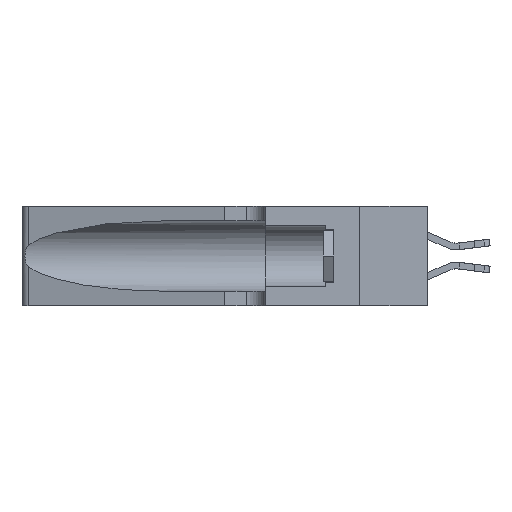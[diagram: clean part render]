
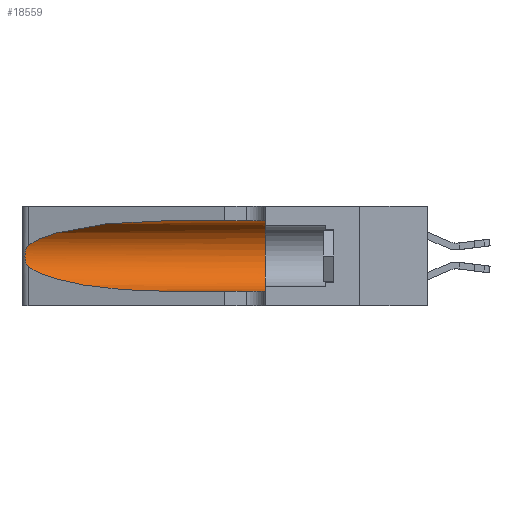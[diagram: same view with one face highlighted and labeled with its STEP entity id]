
A CAD part, left-side view. The second image highlights one B-rep face of the part: STEP entity #18559.
In plain terms, the highlighted cylindrical face has radius 3.308 mm (diameter 6.617 mm), a partial arc.
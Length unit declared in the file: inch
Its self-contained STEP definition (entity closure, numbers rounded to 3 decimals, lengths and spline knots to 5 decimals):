
#207 =( BOUNDED_CURVE ( )  B_SPLINE_CURVE ( 3, ( #34187, #9780, #20865, #4327 ),
 .UNSPECIFIED., .F., .F. ) 
 B_SPLINE_CURVE_WITH_KNOTS ( ( 4, 4 ),
 ( 1.5708, 2.84003 ),
 .UNSPECIFIED. ) 
 CURVE ( )  GEOMETRIC_REPRESENTATION_ITEM ( )  RATIONAL_B_SPLINE_CURVE ( ( 1., 0.87, 0.87, 1. ) ) 
 REPRESENTATION_ITEM ( '' )  );
#319 = LINE ( 'NONE', #3839, #20678 ) ;
#564 = CYLINDRICAL_SURFACE ( 'NONE', #26743, 0.13025 ) ;
#777 = VERTEX_POINT ( 'NONE', #2038 ) ;
#1110 = CARTESIAN_POINT ( 'NONE',  ( 0.26075, 1.23896, 0.19203 ) ) ;
#1728 = EDGE_CURVE ( 'NONE', #10739, #4429, #319, .T. ) ;
#2038 = CARTESIAN_POINT ( 'NONE',  ( 0.25487, 1.22718, 0.14631 ) ) ;
#3839 = CARTESIAN_POINT ( 'NONE',  ( 0.1305, 1.61858, 0.31525 ) ) ;
#3935 = CARTESIAN_POINT ( 'NONE',  ( 0.26017, 1.23833, 0.17102 ) ) ;
#4327 = CARTESIAN_POINT ( 'NONE',  ( 0.25487, 1.22718, 0.22369 ) ) ;
#4376 = CARTESIAN_POINT ( 'NONE',  ( 0.1305, 0.35, 0.05475 ) ) ;
#4429 = VERTEX_POINT ( 'NONE', #34264 ) ;
#4740 = CARTESIAN_POINT ( 'NONE',  ( 0.1305, 0.72297, 0.31525 ) ) ;
#5566 = CIRCLE ( 'NONE', #7672, 0.13025 ) ;
#6512 = DIRECTION ( 'NONE',  ( 0., -1., 0. ) ) ;
#6612 = CARTESIAN_POINT ( 'NONE',  ( 0.25555, 1.22994, 0.2215 ) ) ;
#6734 = CARTESIAN_POINT ( 'NONE',  ( 0.25789, 1.23486, 0.15765 ) ) ;
#7672 = AXIS2_PLACEMENT_3D ( 'NONE', #27172, #10840, #29888 ) ;
#7956 = CARTESIAN_POINT ( 'NONE',  ( 0.1305, 0.72297, 0.05475 ) ) ;
#8739 = VERTEX_POINT ( 'NONE', #25082 ) ;
#9367 = ORIENTED_EDGE ( 'NONE', *, *, #26774, .T. ) ;
#9428 = CARTESIAN_POINT ( 'NONE',  ( 0.1305, 0.72297, 0.05475 ) ) ;
#9519 = CARTESIAN_POINT ( 'NONE',  ( 0.25555, 1.22993, 0.14849 ) ) ;
#9780 = CARTESIAN_POINT ( 'NONE',  ( 0.18966, 0.96281, 0.31525 ) ) ;
#10739 = VERTEX_POINT ( 'NONE', #4740 ) ;
#10840 = DIRECTION ( 'NONE',  ( 0., 1., 0. ) ) ;
#11029 = LINE ( 'NONE', #22103, #25579 ) ;
#11412 = ORIENTED_EDGE ( 'NONE', *, *, #1728, .F. ) ;
#11451 = EDGE_LOOP ( 'NONE', ( #9367, #31678, #34146, #22900, #24126, #11412 ) ) ;
#11585 = DIRECTION ( 'NONE',  ( 0., -1., 0. ) ) ;
#12893 = EDGE_CURVE ( 'NONE', #34045, #18860, #11029, .T. ) ;
#14989 = CARTESIAN_POINT ( 'NONE',  ( 0.25787, 1.23484, 0.2124 ) ) ;
#15813 = B_SPLINE_CURVE_WITH_KNOTS ( 'NONE', 3,
 ( #23095, #6612, #31202, #14989, #33924, #17776, #1110, #20496, #3935, #23217, #6734, #25928, #9519, #28628 ),
 .UNSPECIFIED., .F., .F.,
 ( 4, 2, 2, 2, 2, 2, 4 ),
 ( 0., 0.00027, 0.00053, 0.00107, 0.0016, 0.00187, 0.00214 ),
 .UNSPECIFIED. ) ;
#17146 = CARTESIAN_POINT ( 'NONE',  ( 0.1305, 1.61858, 0.185 ) ) ;
#17776 = CARTESIAN_POINT ( 'NONE',  ( 0.26018, 1.23835, 0.19895 ) ) ;
#18055 = EDGE_CURVE ( 'NONE', #8739, #777, #15813, .T. ) ;
#18559 = ADVANCED_FACE ( 'NONE', ( #22601 ), #564, .F. ) ;
#18860 = VERTEX_POINT ( 'NONE', #4376 ) ;
#18945 = CARTESIAN_POINT ( 'NONE',  ( 0.25487, 1.22718, 0.14631 ) ) ;
#20496 = CARTESIAN_POINT ( 'NONE',  ( 0.26075, 1.23896, 0.178 ) ) ;
#20678 = VECTOR ( 'NONE', #6512, 39.37008 ) ;
#20865 = CARTESIAN_POINT ( 'NONE',  ( 0.2373, 1.15595, 0.28018 ) ) ;
#22103 = CARTESIAN_POINT ( 'NONE',  ( 0.1305, 1.61858, 0.05475 ) ) ;
#22601 = FACE_OUTER_BOUND ( 'NONE', #11451, .T. ) ;
#22900 = ORIENTED_EDGE ( 'NONE', *, *, #12893, .T. ) ;
#23095 = CARTESIAN_POINT ( 'NONE',  ( 0.25487, 1.22718, 0.22369 ) ) ;
#23217 = CARTESIAN_POINT ( 'NONE',  ( 0.25856, 1.23593, 0.16098 ) ) ;
#23756 = EDGE_CURVE ( 'NONE', #777, #34045, #25836, .T. ) ;
#24126 = ORIENTED_EDGE ( 'NONE', *, *, #27734, .F. ) ;
#24384 = CARTESIAN_POINT ( 'NONE',  ( 0.18966, 0.96281, 0.05475 ) ) ;
#25082 = CARTESIAN_POINT ( 'NONE',  ( 0.25487, 1.22718, 0.22369 ) ) ;
#25579 = VECTOR ( 'NONE', #32812, 39.37008 ) ;
#25836 =( BOUNDED_CURVE ( )  B_SPLINE_CURVE ( 3, ( #18945, #35104, #24384, #7956 ),
 .UNSPECIFIED., .F., .F. ) 
 B_SPLINE_CURVE_WITH_KNOTS ( ( 4, 4 ),
 ( 3.44316, 4.71239 ),
 .UNSPECIFIED. ) 
 CURVE ( )  GEOMETRIC_REPRESENTATION_ITEM ( )  RATIONAL_B_SPLINE_CURVE ( ( 1., 0.87, 0.87, 1. ) ) 
 REPRESENTATION_ITEM ( '' )  );
#25928 = CARTESIAN_POINT ( 'NONE',  ( 0.25639, 1.23186, 0.15144 ) ) ;
#26743 = AXIS2_PLACEMENT_3D ( 'NONE', #17146, #11585, #30591 ) ;
#26774 = EDGE_CURVE ( 'NONE', #10739, #8739, #207, .T. ) ;
#27172 = CARTESIAN_POINT ( 'NONE',  ( 0.1305, 0.35, 0.185 ) ) ;
#27734 = EDGE_CURVE ( 'NONE', #4429, #18860, #5566, .T. ) ;
#28628 = CARTESIAN_POINT ( 'NONE',  ( 0.25487, 1.22718, 0.14631 ) ) ;
#29888 = DIRECTION ( 'NONE',  ( 0., 0., 1. ) ) ;
#30591 = DIRECTION ( 'NONE',  ( 0., 0., -1. ) ) ;
#31202 = CARTESIAN_POINT ( 'NONE',  ( 0.25639, 1.23184, 0.21858 ) ) ;
#31678 = ORIENTED_EDGE ( 'NONE', *, *, #18055, .T. ) ;
#32812 = DIRECTION ( 'NONE',  ( 0., -1., 0. ) ) ;
#33924 = CARTESIAN_POINT ( 'NONE',  ( 0.25854, 1.2359, 0.20912 ) ) ;
#34045 = VERTEX_POINT ( 'NONE', #9428 ) ;
#34146 = ORIENTED_EDGE ( 'NONE', *, *, #23756, .T. ) ;
#34187 = CARTESIAN_POINT ( 'NONE',  ( 0.1305, 0.72297, 0.31525 ) ) ;
#34264 = CARTESIAN_POINT ( 'NONE',  ( 0.1305, 0.35, 0.31525 ) ) ;
#35104 = CARTESIAN_POINT ( 'NONE',  ( 0.2373, 1.15595, 0.08982 ) ) ;
